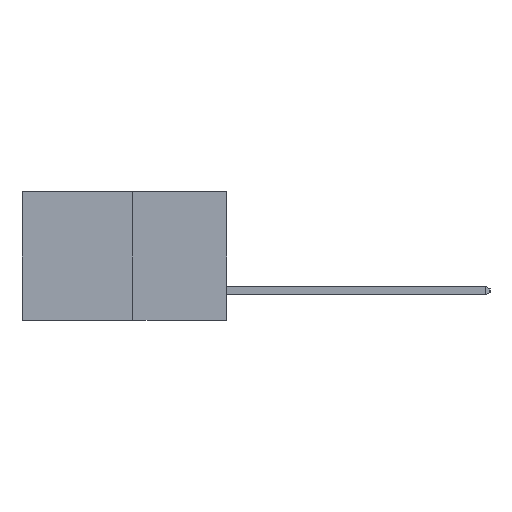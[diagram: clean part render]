
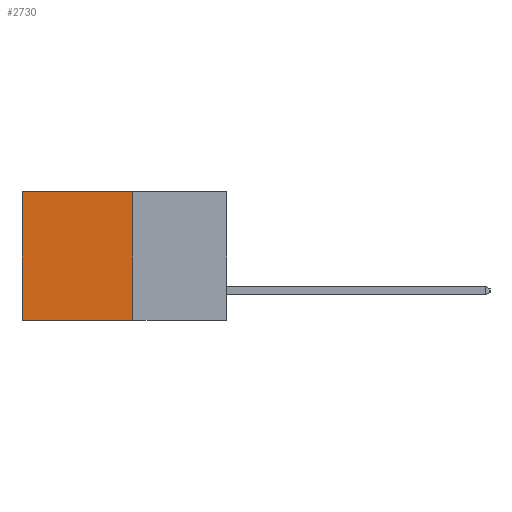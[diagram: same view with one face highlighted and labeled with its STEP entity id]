
A CAD part, left-side view. The second image highlights one B-rep face of the part: STEP entity #2730.
In plain terms, the highlighted planar face has unit normal (-1, 0, 0).
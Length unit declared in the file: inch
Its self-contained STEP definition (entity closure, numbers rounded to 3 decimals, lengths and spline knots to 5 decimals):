
#138 = CARTESIAN_POINT ( 'NONE',  ( 0.277, 0.27, -0.37 ) ) ;
#645 = DIRECTION ( 'NONE',  ( 0., 1., 0. ) ) ;
#765 = ORIENTED_EDGE ( 'NONE', *, *, #2008, .T. ) ;
#834 = CARTESIAN_POINT ( 'NONE',  ( 0.277, 0.27, -0.37 ) ) ;
#1312 = LINE ( 'NONE', #834, #6309 ) ;
#2008 = EDGE_CURVE ( 'NONE', #6288, #8843, #3365, .T. ) ;
#2080 = LINE ( 'NONE', #5916, #4751 ) ;
#2708 = CARTESIAN_POINT ( 'NONE',  ( 0.277, 0.27, 0. ) ) ;
#2730 = ADVANCED_FACE ( 'NONE', ( #9733 ), #4135, .F. ) ;
#3275 = CARTESIAN_POINT ( 'NONE',  ( 0.277, 0.59, -0.37 ) ) ;
#3350 = DIRECTION ( 'NONE',  ( 1., 0., 0. ) ) ;
#3365 = LINE ( 'NONE', #2708, #8598 ) ;
#3998 = EDGE_CURVE ( 'NONE', #8063, #9145, #1312, .T. ) ;
#4135 = PLANE ( 'NONE',  #4864 ) ;
#4359 = CARTESIAN_POINT ( 'NONE',  ( 0.277, 0.27, -0.37 ) ) ;
#4410 = CARTESIAN_POINT ( 'NONE',  ( 0.277, 0.59, 0. ) ) ;
#4751 = VECTOR ( 'NONE', #8803, 39.37008 ) ;
#4864 = AXIS2_PLACEMENT_3D ( 'NONE', #12411, #3350, #10030 ) ;
#4889 = ORIENTED_EDGE ( 'NONE', *, *, #3998, .F. ) ;
#5354 = DIRECTION ( 'NONE',  ( 0., 0., -1. ) ) ;
#5916 = CARTESIAN_POINT ( 'NONE',  ( 0.277, 0.59, -0.37 ) ) ;
#6288 = VERTEX_POINT ( 'NONE', #6832 ) ;
#6309 = VECTOR ( 'NONE', #645, 39.37008 ) ;
#6615 = EDGE_LOOP ( 'NONE', ( #9550, #4889, #7459, #765 ) ) ;
#6693 = EDGE_CURVE ( 'NONE', #6288, #8063, #8926, .T. ) ;
#6832 = CARTESIAN_POINT ( 'NONE',  ( 0.277, 0.27, 0. ) ) ;
#7459 = ORIENTED_EDGE ( 'NONE', *, *, #6693, .F. ) ;
#8063 = VERTEX_POINT ( 'NONE', #138 ) ;
#8598 = VECTOR ( 'NONE', #8689, 39.37008 ) ;
#8689 = DIRECTION ( 'NONE',  ( 0., 1., 0. ) ) ;
#8803 = DIRECTION ( 'NONE',  ( 0., 0., -1. ) ) ;
#8843 = VERTEX_POINT ( 'NONE', #4410 ) ;
#8926 = LINE ( 'NONE', #4359, #11092 ) ;
#9145 = VERTEX_POINT ( 'NONE', #3275 ) ;
#9550 = ORIENTED_EDGE ( 'NONE', *, *, #11343, .T. ) ;
#9733 = FACE_OUTER_BOUND ( 'NONE', #6615, .T. ) ;
#10030 = DIRECTION ( 'NONE',  ( 0., 0., -1. ) ) ;
#11092 = VECTOR ( 'NONE', #5354, 39.37008 ) ;
#11343 = EDGE_CURVE ( 'NONE', #8843, #9145, #2080, .T. ) ;
#12411 = CARTESIAN_POINT ( 'NONE',  ( 0.277, 0.27, -0.37 ) ) ;
